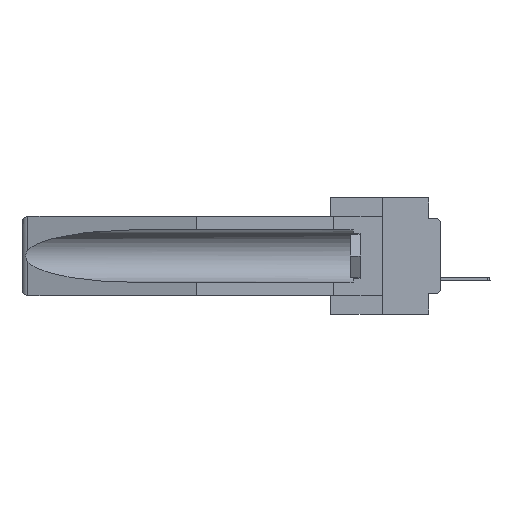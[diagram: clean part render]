
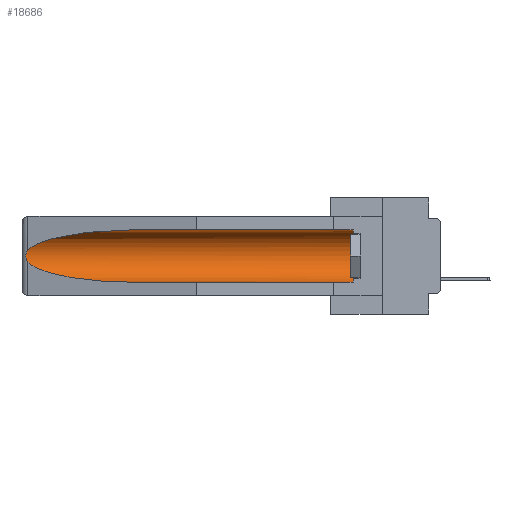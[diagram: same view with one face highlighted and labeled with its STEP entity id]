
A CAD part, left-side view. The second image highlights one B-rep face of the part: STEP entity #18686.
In plain terms, the highlighted cylindrical face has radius 2.857 mm (diameter 5.715 mm), a partial arc.
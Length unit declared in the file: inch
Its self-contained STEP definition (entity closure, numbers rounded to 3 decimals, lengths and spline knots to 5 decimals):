
#1788 = CARTESIAN_POINT ( 'NONE',  ( 0.26537, 1.52718, -0.19328 ) ) ;
#1818 = VERTEX_POINT ( 'NONE', #24636 ) ;
#1961 = CARTESIAN_POINT ( 'NONE',  ( 0.26537, 1.52718, -0.14972 ) ) ;
#2033 = ORIENTED_EDGE ( 'NONE', *, *, #34879, .T. ) ;
#2420 =( BOUNDED_CURVE ( )  B_SPLINE_CURVE ( 3, ( #29652, #14285, #14643, #17431 ),
 .UNSPECIFIED., .F., .F. ) 
 B_SPLINE_CURVE_WITH_KNOTS ( ( 4, 4 ),
 ( 4.71239, 6.08839 ),
 .UNSPECIFIED. ) 
 CURVE ( )  GEOMETRIC_REPRESENTATION_ITEM ( )  RATIONAL_B_SPLINE_CURVE ( ( 1., 0.848, 0.848, 1. ) ) 
 REPRESENTATION_ITEM ( '' )  );
#2819 = CARTESIAN_POINT ( 'NONE',  ( 0.26597, 1.5296, -0.19026 ) ) ;
#3493 = AXIS2_PLACEMENT_3D ( 'NONE', #28603, #31347, #34126 ) ;
#4664 = CARTESIAN_POINT ( 'NONE',  ( 0.155, -0.30754, -0.284 ) ) ;
#5093 = ORIENTED_EDGE ( 'NONE', *, *, #11079, .T. ) ;
#5453 = ORIENTED_EDGE ( 'NONE', *, *, #16250, .F. ) ;
#5665 =( BOUNDED_CURVE ( )  B_SPLINE_CURVE ( 3, ( #1788, #7260, #20796, #26189 ),
 .UNSPECIFIED., .F., .F. ) 
 B_SPLINE_CURVE_WITH_KNOTS ( ( 4, 4 ),
 ( 0.1948, 1.5708 ),
 .UNSPECIFIED. ) 
 CURVE ( )  GEOMETRIC_REPRESENTATION_ITEM ( )  RATIONAL_B_SPLINE_CURVE ( ( 1., 0.848, 0.848, 1. ) ) 
 REPRESENTATION_ITEM ( '' )  );
#6282 = CARTESIAN_POINT ( 'NONE',  ( 0.155, 0.126, -0.1715 ) ) ;
#6541 = CARTESIAN_POINT ( 'NONE',  ( 0.26597, 1.52961, -0.15275 ) ) ;
#6653 = CARTESIAN_POINT ( 'NONE',  ( 0.26537, 1.52718, -0.14972 ) ) ;
#7024 = VERTEX_POINT ( 'NONE', #35473 ) ;
#7260 = CARTESIAN_POINT ( 'NONE',  ( 0.25451, 1.48313, -0.24835 ) ) ;
#7955 = CIRCLE ( 'NONE', #25862, 0.1125 ) ;
#9157 = DIRECTION ( 'NONE',  ( 0., 1., 0. ) ) ;
#9286 = CARTESIAN_POINT ( 'NONE',  ( 0.26654, 1.53092, -0.15636 ) ) ;
#9556 = EDGE_LOOP ( 'NONE', ( #5093, #31774, #24173, #5453, #18369, #2033 ) ) ;
#9775 = CYLINDRICAL_SURFACE ( 'NONE', #3493, 0.1125 ) ;
#10266 = VERTEX_POINT ( 'NONE', #1961 ) ;
#11079 = EDGE_CURVE ( 'NONE', #7024, #10266, #2420, .T. ) ;
#11391 = CARTESIAN_POINT ( 'NONE',  ( 0.2673, 1.53269, -0.17917 ) ) ;
#11769 = VERTEX_POINT ( 'NONE', #33492 ) ;
#12452 = EDGE_CURVE ( 'NONE', #10266, #1818, #14224, .T. ) ;
#12703 = VERTEX_POINT ( 'NONE', #34840 ) ;
#13163 = DIRECTION ( 'NONE',  ( 0., 1., 0. ) ) ;
#14224 = B_SPLINE_CURVE_WITH_KNOTS ( 'NONE', 3,
 ( #6653, #6541, #9286, #28479, #14642, #15483, #11391, #33452, #2819, #19211 ),
 .UNSPECIFIED., .F., .F.,
 ( 4, 2, 2, 2, 4 ),
 ( 0., 0.00029, 0.00058, 0.00087, 0.00117 ),
 .UNSPECIFIED. ) ;
#14285 = CARTESIAN_POINT ( 'NONE',  ( 0.21114, 1.30732, -0.059 ) ) ;
#14642 = CARTESIAN_POINT ( 'NONE',  ( 0.2675, 1.53308, -0.16763 ) ) ;
#14643 = CARTESIAN_POINT ( 'NONE',  ( 0.25451, 1.48313, -0.09465 ) ) ;
#14694 = DIRECTION ( 'NONE',  ( 0., 0., 1. ) ) ;
#15483 = CARTESIAN_POINT ( 'NONE',  ( 0.2675, 1.53308, -0.17534 ) ) ;
#16250 = EDGE_CURVE ( 'NONE', #34874, #11769, #25425, .T. ) ;
#17431 = CARTESIAN_POINT ( 'NONE',  ( 0.26537, 1.52718, -0.14972 ) ) ;
#18369 = ORIENTED_EDGE ( 'NONE', *, *, #31446, .T. ) ;
#18686 = ADVANCED_FACE ( 'NONE', ( #35114 ), #9775, .F. ) ;
#18820 = EDGE_CURVE ( 'NONE', #1818, #11769, #5665, .T. ) ;
#19211 = CARTESIAN_POINT ( 'NONE',  ( 0.26537, 1.52718, -0.19328 ) ) ;
#20066 = DIRECTION ( 'NONE',  ( 0., -1., 0. ) ) ;
#20796 = CARTESIAN_POINT ( 'NONE',  ( 0.21114, 1.30732, -0.284 ) ) ;
#23655 = LINE ( 'NONE', #28237, #29717 ) ;
#23702 = VECTOR ( 'NONE', #13163, 39.37008 ) ;
#24173 = ORIENTED_EDGE ( 'NONE', *, *, #18820, .T. ) ;
#24636 = CARTESIAN_POINT ( 'NONE',  ( 0.26537, 1.52718, -0.19328 ) ) ;
#25425 = LINE ( 'NONE', #4664, #23702 ) ;
#25862 = AXIS2_PLACEMENT_3D ( 'NONE', #6282, #20066, #14694 ) ;
#26189 = CARTESIAN_POINT ( 'NONE',  ( 0.155, 1.07973, -0.284 ) ) ;
#28237 = CARTESIAN_POINT ( 'NONE',  ( 0.155, -0.30754, -0.059 ) ) ;
#28479 = CARTESIAN_POINT ( 'NONE',  ( 0.2673, 1.5327, -0.16383 ) ) ;
#28603 = CARTESIAN_POINT ( 'NONE',  ( 0.155, -0.30754, -0.1715 ) ) ;
#29652 = CARTESIAN_POINT ( 'NONE',  ( 0.155, 1.07973, -0.059 ) ) ;
#29717 = VECTOR ( 'NONE', #9157, 39.37008 ) ;
#31347 = DIRECTION ( 'NONE',  ( 0., 1., 0. ) ) ;
#31446 = EDGE_CURVE ( 'NONE', #34874, #12703, #7955, .T. ) ;
#31774 = ORIENTED_EDGE ( 'NONE', *, *, #12452, .T. ) ;
#33452 = CARTESIAN_POINT ( 'NONE',  ( 0.26655, 1.53094, -0.18657 ) ) ;
#33492 = CARTESIAN_POINT ( 'NONE',  ( 0.155, 1.07973, -0.284 ) ) ;
#33643 = CARTESIAN_POINT ( 'NONE',  ( 0.155, 0.126, -0.284 ) ) ;
#34126 = DIRECTION ( 'NONE',  ( 0., 0., 1. ) ) ;
#34840 = CARTESIAN_POINT ( 'NONE',  ( 0.155, 0.126, -0.059 ) ) ;
#34874 = VERTEX_POINT ( 'NONE', #33643 ) ;
#34879 = EDGE_CURVE ( 'NONE', #12703, #7024, #23655, .T. ) ;
#35114 = FACE_OUTER_BOUND ( 'NONE', #9556, .T. ) ;
#35473 = CARTESIAN_POINT ( 'NONE',  ( 0.155, 1.07973, -0.059 ) ) ;
